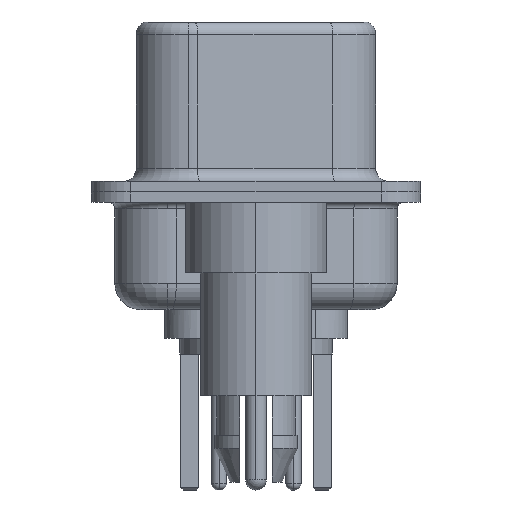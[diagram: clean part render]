
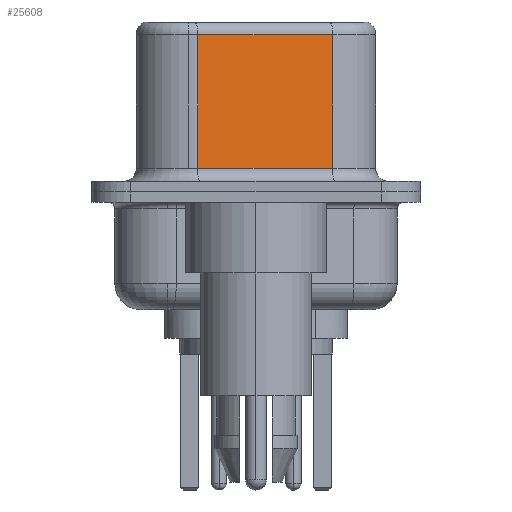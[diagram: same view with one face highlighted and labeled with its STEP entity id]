
A CAD part, left-side view. The second image highlights one B-rep face of the part: STEP entity #25608.
In plain terms, the highlighted planar face has unit normal (-0.985, -0.174, 0).
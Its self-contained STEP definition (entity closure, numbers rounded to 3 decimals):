
#879 = EDGE_CURVE ( 'NONE', #1405, #15038, #4568, .T. ) ;
#1405 = VERTEX_POINT ( 'NONE', #20182 ) ;
#1446 = EDGE_CURVE ( 'NONE', #25518, #8699, #13022, .T. ) ;
#2188 = DIRECTION ( 'NONE',  ( -0.174, 0.985, 0. ) ) ;
#2261 = VECTOR ( 'NONE', #2188, 1000. ) ;
#2566 = DIRECTION ( 'NONE',  ( 0.985, 0.174, 0. ) ) ;
#3687 = LINE ( 'NONE', #25091, #14520 ) ;
#4406 = CARTESIAN_POINT ( 'NONE',  ( 4.585, -2.927, 6.02 ) ) ;
#4568 = LINE ( 'NONE', #4406, #2261 ) ;
#5009 = CARTESIAN_POINT ( 'NONE',  ( 3.675, 2.233, 6.02 ) ) ;
#5672 = LINE ( 'NONE', #13403, #20091 ) ;
#6420 = CARTESIAN_POINT ( 'NONE',  ( 3.675, 2.233, 0.9 ) ) ;
#6721 = AXIS2_PLACEMENT_3D ( 'NONE', #8710, #2566, #21236 ) ;
#7656 = ORIENTED_EDGE ( 'NONE', *, *, #21087, .T. ) ;
#8100 = EDGE_LOOP ( 'NONE', ( #22216, #13593, #7656, #13822 ) ) ;
#8699 = VERTEX_POINT ( 'NONE', #15045 ) ;
#8710 = CARTESIAN_POINT ( 'NONE',  ( 4.585, -2.927, 6.52 ) ) ;
#9821 = DIRECTION ( 'NONE',  ( 0.174, -0.985, 0. ) ) ;
#10899 = FACE_OUTER_BOUND ( 'NONE', #8100, .T. ) ;
#13022 = LINE ( 'NONE', #16350, #14015 ) ;
#13403 = CARTESIAN_POINT ( 'NONE',  ( 3.675, 2.233, 6.52 ) ) ;
#13593 = ORIENTED_EDGE ( 'NONE', *, *, #879, .T. ) ;
#13822 = ORIENTED_EDGE ( 'NONE', *, *, #1446, .T. ) ;
#14015 = VECTOR ( 'NONE', #9821, 1000. ) ;
#14520 = VECTOR ( 'NONE', #18731, 1000. ) ;
#15038 = VERTEX_POINT ( 'NONE', #5009 ) ;
#15045 = CARTESIAN_POINT ( 'NONE',  ( 4.585, -2.927, 0.9 ) ) ;
#16350 = CARTESIAN_POINT ( 'NONE',  ( 4.585, -2.927, 0.9 ) ) ;
#18731 = DIRECTION ( 'NONE',  ( 0., 0., -1. ) ) ;
#19578 = DIRECTION ( 'NONE',  ( 0., 0., -1. ) ) ;
#20091 = VECTOR ( 'NONE', #19578, 1000. ) ;
#20182 = CARTESIAN_POINT ( 'NONE',  ( 4.585, -2.927, 6.02 ) ) ;
#21087 = EDGE_CURVE ( 'NONE', #15038, #25518, #5672, .T. ) ;
#21236 = DIRECTION ( 'NONE',  ( -0.174, 0.985, 0. ) ) ;
#22094 = EDGE_CURVE ( 'NONE', #1405, #8699, #3687, .T. ) ;
#22216 = ORIENTED_EDGE ( 'NONE', *, *, #22094, .F. ) ;
#23430 = PLANE ( 'NONE',  #6721 ) ;
#25091 = CARTESIAN_POINT ( 'NONE',  ( 4.585, -2.927, 6.52 ) ) ;
#25518 = VERTEX_POINT ( 'NONE', #6420 ) ;
#25608 = ADVANCED_FACE ( 'NONE', ( #10899 ), #23430, .F. ) ;
